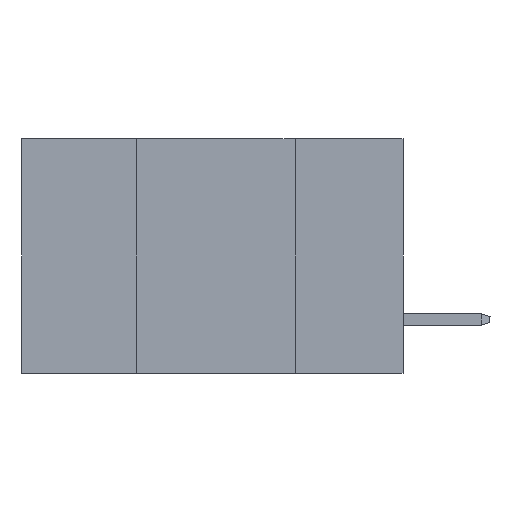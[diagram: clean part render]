
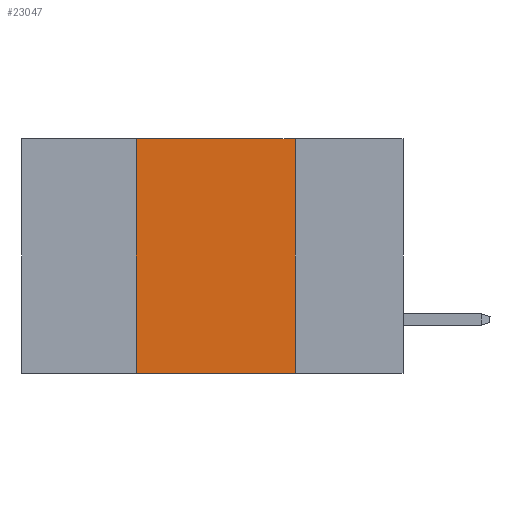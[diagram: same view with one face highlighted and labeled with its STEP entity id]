
A CAD part, left-side view. The second image highlights one B-rep face of the part: STEP entity #23047.
In plain terms, the highlighted planar face has unit normal (-1, 0, 0).
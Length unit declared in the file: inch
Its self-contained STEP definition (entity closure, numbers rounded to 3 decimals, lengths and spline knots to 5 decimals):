
#628 = CARTESIAN_POINT ( 'NONE',  ( 0., 0.17, 0. ) ) ;
#1550 = EDGE_CURVE ( 'NONE', #13455, #16667, #25941, .T. ) ;
#2328 = EDGE_LOOP ( 'NONE', ( #7366, #17342, #2788, #20440 ) ) ;
#2570 = AXIS2_PLACEMENT_3D ( 'NONE', #6280, #22862, #21102 ) ;
#2788 = ORIENTED_EDGE ( 'NONE', *, *, #1550, .F. ) ;
#3311 = EDGE_CURVE ( 'NONE', #16667, #22785, #15140, .T. ) ;
#6280 = CARTESIAN_POINT ( 'NONE',  ( 0., 0.6, 0. ) ) ;
#6449 = VECTOR ( 'NONE', #11561, 39.37008 ) ;
#6878 = EDGE_CURVE ( 'NONE', #22785, #8554, #21045, .T. ) ;
#7366 = ORIENTED_EDGE ( 'NONE', *, *, #6878, .F. ) ;
#7479 = CARTESIAN_POINT ( 'NONE',  ( 0., 0.42, 0. ) ) ;
#7917 = CARTESIAN_POINT ( 'NONE',  ( 0., 0.42, -0.37 ) ) ;
#7995 = VECTOR ( 'NONE', #23208, 39.37008 ) ;
#8308 = CARTESIAN_POINT ( 'NONE',  ( 0., 0.42, 0. ) ) ;
#8554 = VERTEX_POINT ( 'NONE', #12584 ) ;
#9247 = VECTOR ( 'NONE', #19462, 39.37008 ) ;
#10856 = CARTESIAN_POINT ( 'NONE',  ( 0., 0.6, -0.37 ) ) ;
#11561 = DIRECTION ( 'NONE',  ( 0., 0., 1. ) ) ;
#12402 = FACE_OUTER_BOUND ( 'NONE', #2328, .T. ) ;
#12584 = CARTESIAN_POINT ( 'NONE',  ( 0., 0.17, -0.37 ) ) ;
#12757 = DIRECTION ( 'NONE',  ( 0., -1., 0. ) ) ;
#13455 = VERTEX_POINT ( 'NONE', #7917 ) ;
#14719 = PLANE ( 'NONE',  #2570 ) ;
#15140 = LINE ( 'NONE', #23393, #9247 ) ;
#16667 = VERTEX_POINT ( 'NONE', #8308 ) ;
#17200 = EDGE_CURVE ( 'NONE', #13455, #8554, #21059, .T. ) ;
#17342 = ORIENTED_EDGE ( 'NONE', *, *, #3311, .F. ) ;
#19462 = DIRECTION ( 'NONE',  ( 0., -1., 0. ) ) ;
#20440 = ORIENTED_EDGE ( 'NONE', *, *, #17200, .T. ) ;
#21045 = LINE ( 'NONE', #628, #7995 ) ;
#21059 = LINE ( 'NONE', #10856, #21468 ) ;
#21102 = DIRECTION ( 'NONE',  ( 0., 0., -1. ) ) ;
#21468 = VECTOR ( 'NONE', #12757, 39.37008 ) ;
#21803 = CARTESIAN_POINT ( 'NONE',  ( 0., 0.17, 0. ) ) ;
#22785 = VERTEX_POINT ( 'NONE', #21803 ) ;
#22862 = DIRECTION ( 'NONE',  ( 1., 0., 0. ) ) ;
#23047 = ADVANCED_FACE ( 'NONE', ( #12402 ), #14719, .F. ) ;
#23208 = DIRECTION ( 'NONE',  ( 0., 0., -1. ) ) ;
#23393 = CARTESIAN_POINT ( 'NONE',  ( 0., 0.6, 0. ) ) ;
#25941 = LINE ( 'NONE', #7479, #6449 ) ;
